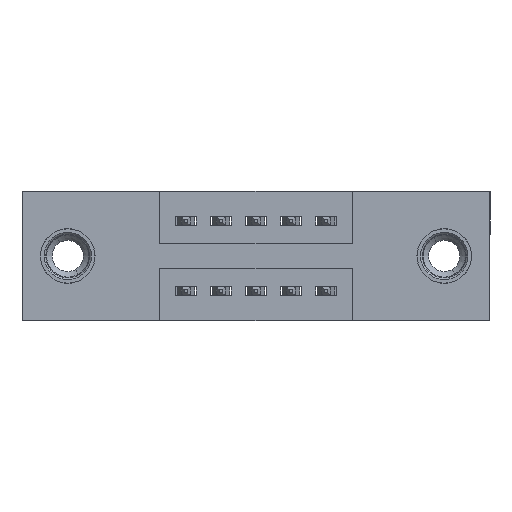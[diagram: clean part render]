
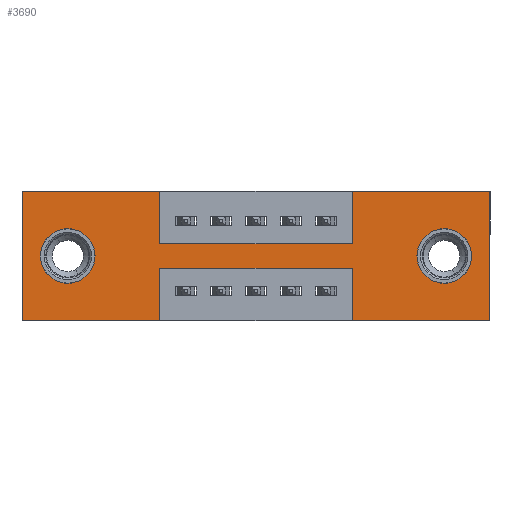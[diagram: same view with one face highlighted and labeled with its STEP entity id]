
A CAD part, front view. The second image highlights one B-rep face of the part: STEP entity #3690.
In plain terms, the highlighted planar face has unit normal (0, -1, 0).
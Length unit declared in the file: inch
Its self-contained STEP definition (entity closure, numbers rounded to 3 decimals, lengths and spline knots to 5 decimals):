
#179 = CARTESIAN_POINT ( 'NONE',  ( 1.335, 0., 0. ) ) ;
#256 = VERTEX_POINT ( 'NONE', #13589 ) ;
#450 = ORIENTED_EDGE ( 'NONE', *, *, #11146, .T. ) ;
#451 = DIRECTION ( 'NONE',  ( -1., 0., 0. ) ) ;
#457 = DIRECTION ( 'NONE',  ( 0., 0., 1. ) ) ;
#460 = VERTEX_POINT ( 'NONE', #3734 ) ;
#524 = AXIS2_PLACEMENT_3D ( 'NONE', #11794, #12859, #1402 ) ;
#546 = EDGE_CURVE ( 'NONE', #1991, #256, #2931, .T. ) ;
#604 = CIRCLE ( 'NONE', #697, 0.078 ) ;
#658 = ORIENTED_EDGE ( 'NONE', *, *, #546, .F. ) ;
#697 = AXIS2_PLACEMENT_3D ( 'NONE', #4680, #6892, #4857 ) ;
#706 = CARTESIAN_POINT ( 'NONE',  ( 0.13, 0., -0.185 ) ) ;
#742 = DIRECTION ( 'NONE',  ( 0., 0., 1. ) ) ;
#1087 = LINE ( 'NONE', #10497, #6052 ) ;
#1089 = LINE ( 'NONE', #1694, #11847 ) ;
#1384 = EDGE_CURVE ( 'NONE', #460, #2157, #6889, .T. ) ;
#1385 = CARTESIAN_POINT ( 'NONE',  ( 1.335, 0., 0. ) ) ;
#1402 = DIRECTION ( 'NONE',  ( 0., 0., -1. ) ) ;
#1526 = EDGE_CURVE ( 'NONE', #1849, #12489, #7044, .T. ) ;
#1625 = EDGE_CURVE ( 'NONE', #7911, #7828, #2888, .T. ) ;
#1694 = CARTESIAN_POINT ( 'NONE',  ( 0., 0., 0. ) ) ;
#1830 = AXIS2_PLACEMENT_3D ( 'NONE', #2040, #6289, #3101 ) ;
#1849 = VERTEX_POINT ( 'NONE', #12468 ) ;
#1874 = LINE ( 'NONE', #7361, #3377 ) ;
#1906 = DIRECTION ( 'NONE',  ( 0., 0., 1. ) ) ;
#1949 = DIRECTION ( 'NONE',  ( 1., 0., 0. ) ) ;
#1991 = VERTEX_POINT ( 'NONE', #11530 ) ;
#2040 = CARTESIAN_POINT ( 'NONE',  ( 1.205, 0., -0.185 ) ) ;
#2157 = VERTEX_POINT ( 'NONE', #6903 ) ;
#2194 = VERTEX_POINT ( 'NONE', #10640 ) ;
#2396 = VECTOR ( 'NONE', #2710, 39.37008 ) ;
#2441 = VECTOR ( 'NONE', #742, 39.37008 ) ;
#2534 = VERTEX_POINT ( 'NONE', #13643 ) ;
#2623 = EDGE_CURVE ( 'NONE', #12662, #11368, #7626, .T. ) ;
#2710 = DIRECTION ( 'NONE',  ( 0., 0., -1. ) ) ;
#2788 = FACE_OUTER_BOUND ( 'NONE', #9976, .T. ) ;
#2888 = LINE ( 'NONE', #3213, #7705 ) ;
#2931 = LINE ( 'NONE', #12045, #4097 ) ;
#2981 = VECTOR ( 'NONE', #11593, 39.37008 ) ;
#3019 = DIRECTION ( 'NONE',  ( 0., 0., 1. ) ) ;
#3067 = VECTOR ( 'NONE', #3538, 39.37008 ) ;
#3101 = DIRECTION ( 'NONE',  ( 0., 0., -1. ) ) ;
#3213 = CARTESIAN_POINT ( 'NONE',  ( 0.9425, 0., 0. ) ) ;
#3227 = CARTESIAN_POINT ( 'NONE',  ( 0.9425, 0., -0.22 ) ) ;
#3292 = ORIENTED_EDGE ( 'NONE', *, *, #13432, .F. ) ;
#3342 = DIRECTION ( 'NONE',  ( 0., 0., -1. ) ) ;
#3355 = LINE ( 'NONE', #179, #7811 ) ;
#3377 = VECTOR ( 'NONE', #7413, 39.37008 ) ;
#3487 = CARTESIAN_POINT ( 'NONE',  ( 0.3925, 0., 0. ) ) ;
#3538 = DIRECTION ( 'NONE',  ( 0., 0., -1. ) ) ;
#3690 = ADVANCED_FACE ( 'NONE', ( #10559, #4288, #2788 ), #10830, .T. ) ;
#3734 = CARTESIAN_POINT ( 'NONE',  ( 0., 0., -0.37 ) ) ;
#4097 = VECTOR ( 'NONE', #451, 39.37008 ) ;
#4116 = ORIENTED_EDGE ( 'NONE', *, *, #5170, .F. ) ;
#4288 = FACE_BOUND ( 'NONE', #5889, .T. ) ;
#4357 = VERTEX_POINT ( 'NONE', #6580 ) ;
#4426 = EDGE_CURVE ( 'NONE', #4357, #8818, #604, .T. ) ;
#4680 = CARTESIAN_POINT ( 'NONE',  ( 1.205, 0., -0.185 ) ) ;
#4746 = CARTESIAN_POINT ( 'NONE',  ( 0.9425, 0., -0.37 ) ) ;
#4857 = DIRECTION ( 'NONE',  ( 0., 0., -1. ) ) ;
#4929 = DIRECTION ( 'NONE',  ( -1., 0., 0. ) ) ;
#5019 = CARTESIAN_POINT ( 'NONE',  ( 1.205, 0., -0.107 ) ) ;
#5035 = VERTEX_POINT ( 'NONE', #1385 ) ;
#5041 = ORIENTED_EDGE ( 'NONE', *, *, #1526, .T. ) ;
#5126 = ORIENTED_EDGE ( 'NONE', *, *, #10948, .T. ) ;
#5170 = EDGE_CURVE ( 'NONE', #2157, #5436, #1089, .T. ) ;
#5436 = VERTEX_POINT ( 'NONE', #6412 ) ;
#5611 = CARTESIAN_POINT ( 'NONE',  ( 0.9425, 0., -0.15 ) ) ;
#5764 = LINE ( 'NONE', #4746, #11344 ) ;
#5773 = CARTESIAN_POINT ( 'NONE',  ( 0.3925, 0., -0.37 ) ) ;
#5863 = CARTESIAN_POINT ( 'NONE',  ( 0.13, 0., -0.263 ) ) ;
#5889 = EDGE_LOOP ( 'NONE', ( #5041, #5126 ) ) ;
#5900 = CARTESIAN_POINT ( 'NONE',  ( 0., 0., -0.37 ) ) ;
#5947 = DIRECTION ( 'NONE',  ( 1., 0., 0. ) ) ;
#6052 = VECTOR ( 'NONE', #1949, 39.37008 ) ;
#6131 = ORIENTED_EDGE ( 'NONE', *, *, #9062, .F. ) ;
#6246 = ORIENTED_EDGE ( 'NONE', *, *, #7749, .F. ) ;
#6289 = DIRECTION ( 'NONE',  ( 0., 1., 0. ) ) ;
#6412 = CARTESIAN_POINT ( 'NONE',  ( 0.3925, 0., 0. ) ) ;
#6486 = ORIENTED_EDGE ( 'NONE', *, *, #1384, .F. ) ;
#6580 = CARTESIAN_POINT ( 'NONE',  ( 1.205, 0., -0.263 ) ) ;
#6739 = DIRECTION ( 'NONE',  ( 0., 0., 1. ) ) ;
#6847 = CARTESIAN_POINT ( 'NONE',  ( 0.13, 0., -0.185 ) ) ;
#6889 = LINE ( 'NONE', #6956, #2441 ) ;
#6892 = DIRECTION ( 'NONE',  ( 0., 1., 0. ) ) ;
#6903 = CARTESIAN_POINT ( 'NONE',  ( 0., 0., 0. ) ) ;
#6956 = CARTESIAN_POINT ( 'NONE',  ( 0., 0., 0. ) ) ;
#7044 = CIRCLE ( 'NONE', #12283, 0.078 ) ;
#7178 = ORIENTED_EDGE ( 'NONE', *, *, #13172, .F. ) ;
#7254 = CIRCLE ( 'NONE', #1830, 0.078 ) ;
#7361 = CARTESIAN_POINT ( 'NONE',  ( 0.3925, 0., -0.15 ) ) ;
#7413 = DIRECTION ( 'NONE',  ( 1., 0., 0. ) ) ;
#7557 = EDGE_CURVE ( 'NONE', #11368, #2194, #10482, .T. ) ;
#7591 = CIRCLE ( 'NONE', #8650, 0.078 ) ;
#7626 = LINE ( 'NONE', #9475, #2981 ) ;
#7705 = VECTOR ( 'NONE', #3019, 39.37008 ) ;
#7749 = EDGE_CURVE ( 'NONE', #2534, #7911, #1874, .T. ) ;
#7811 = VECTOR ( 'NONE', #3342, 39.37008 ) ;
#7828 = VERTEX_POINT ( 'NONE', #8696 ) ;
#7911 = VERTEX_POINT ( 'NONE', #5611 ) ;
#7934 = CARTESIAN_POINT ( 'NONE',  ( 0.3925, 0., -0.22 ) ) ;
#8437 = EDGE_CURVE ( 'NONE', #5035, #1991, #3355, .T. ) ;
#8650 = AXIS2_PLACEMENT_3D ( 'NONE', #6847, #13076, #457 ) ;
#8662 = ORIENTED_EDGE ( 'NONE', *, *, #8437, .F. ) ;
#8696 = CARTESIAN_POINT ( 'NONE',  ( 0.9425, 0., 0. ) ) ;
#8818 = VERTEX_POINT ( 'NONE', #5019 ) ;
#9062 = EDGE_CURVE ( 'NONE', #256, #12662, #5764, .T. ) ;
#9475 = CARTESIAN_POINT ( 'NONE',  ( 0.3925, 0., -0.22 ) ) ;
#9761 = LINE ( 'NONE', #5900, #10419 ) ;
#9776 = EDGE_CURVE ( 'NONE', #2194, #460, #9761, .T. ) ;
#9976 = EDGE_LOOP ( 'NONE', ( #13511, #11270, #6131, #658, #8662, #7178, #12166, #6246, #3292, #4116, #6486, #11749 ) ) ;
#10319 = ORIENTED_EDGE ( 'NONE', *, *, #4426, .T. ) ;
#10419 = VECTOR ( 'NONE', #4929, 39.37008 ) ;
#10482 = LINE ( 'NONE', #5773, #2396 ) ;
#10497 = CARTESIAN_POINT ( 'NONE',  ( 0., 0., 0. ) ) ;
#10559 = FACE_BOUND ( 'NONE', #11424, .T. ) ;
#10640 = CARTESIAN_POINT ( 'NONE',  ( 0.3925, 0., -0.37 ) ) ;
#10830 = PLANE ( 'NONE',  #524 ) ;
#10948 = EDGE_CURVE ( 'NONE', #12489, #1849, #7591, .T. ) ;
#11020 = LINE ( 'NONE', #3487, #3067 ) ;
#11146 = EDGE_CURVE ( 'NONE', #8818, #4357, #7254, .T. ) ;
#11270 = ORIENTED_EDGE ( 'NONE', *, *, #2623, .F. ) ;
#11344 = VECTOR ( 'NONE', #6739, 39.37008 ) ;
#11368 = VERTEX_POINT ( 'NONE', #7934 ) ;
#11424 = EDGE_LOOP ( 'NONE', ( #450, #10319 ) ) ;
#11530 = CARTESIAN_POINT ( 'NONE',  ( 1.335, 0., -0.37 ) ) ;
#11593 = DIRECTION ( 'NONE',  ( -1., 0., 0. ) ) ;
#11749 = ORIENTED_EDGE ( 'NONE', *, *, #9776, .F. ) ;
#11794 = CARTESIAN_POINT ( 'NONE',  ( 0., 0., -0.37 ) ) ;
#11847 = VECTOR ( 'NONE', #5947, 39.37008 ) ;
#12045 = CARTESIAN_POINT ( 'NONE',  ( 0., 0., -0.37 ) ) ;
#12166 = ORIENTED_EDGE ( 'NONE', *, *, #1625, .F. ) ;
#12283 = AXIS2_PLACEMENT_3D ( 'NONE', #706, #12440, #1906 ) ;
#12440 = DIRECTION ( 'NONE',  ( 0., 1., 0. ) ) ;
#12468 = CARTESIAN_POINT ( 'NONE',  ( 0.13, 0., -0.107 ) ) ;
#12489 = VERTEX_POINT ( 'NONE', #5863 ) ;
#12662 = VERTEX_POINT ( 'NONE', #3227 ) ;
#12859 = DIRECTION ( 'NONE',  ( 0., -1., 0. ) ) ;
#13076 = DIRECTION ( 'NONE',  ( 0., 1., 0. ) ) ;
#13172 = EDGE_CURVE ( 'NONE', #7828, #5035, #1087, .T. ) ;
#13432 = EDGE_CURVE ( 'NONE', #5436, #2534, #11020, .T. ) ;
#13511 = ORIENTED_EDGE ( 'NONE', *, *, #7557, .F. ) ;
#13589 = CARTESIAN_POINT ( 'NONE',  ( 0.9425, 0., -0.37 ) ) ;
#13643 = CARTESIAN_POINT ( 'NONE',  ( 0.3925, 0., -0.15 ) ) ;
